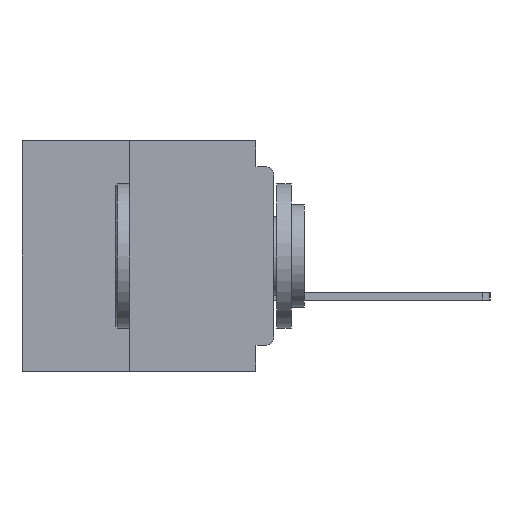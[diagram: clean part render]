
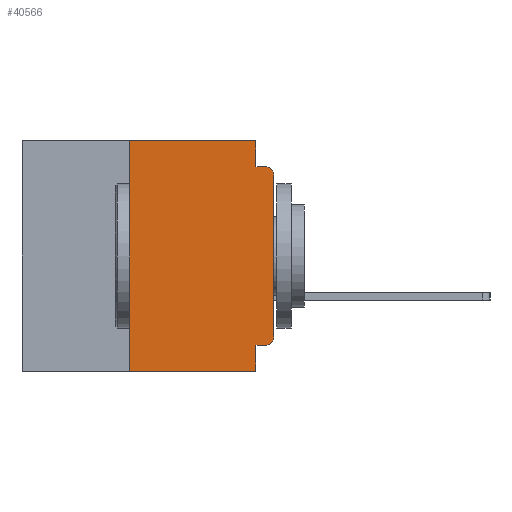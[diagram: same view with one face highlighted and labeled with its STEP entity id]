
A CAD part, left-side view. The second image highlights one B-rep face of the part: STEP entity #40566.
In plain terms, the highlighted planar face has unit normal (-1, 0, 0).
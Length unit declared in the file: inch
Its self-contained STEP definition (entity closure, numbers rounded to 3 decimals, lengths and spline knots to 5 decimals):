
#338 = VECTOR ( 'NONE', #13728, 39.37008 ) ;
#864 = CARTESIAN_POINT ( 'NONE',  ( 0., 0.015, -0.06 ) ) ;
#942 = FACE_OUTER_BOUND ( 'NONE', #18045, .T. ) ;
#963 = EDGE_CURVE ( 'NONE', #47826, #32119, #23893, .T. ) ;
#2531 = CARTESIAN_POINT ( 'NONE',  ( 0., 0.437, -0.4 ) ) ;
#3249 = VECTOR ( 'NONE', #39282, 39.37008 ) ;
#3301 = DIRECTION ( 'NONE',  ( -1., 0., 0. ) ) ;
#3614 = VECTOR ( 'NONE', #4385, 39.37008 ) ;
#4385 = DIRECTION ( 'NONE',  ( 0., 0., 1. ) ) ;
#4630 = LINE ( 'NONE', #17301, #3249 ) ;
#5365 = DIRECTION ( 'NONE',  ( 0., 0., -1. ) ) ;
#6718 = DIRECTION ( 'NONE',  ( 0., 0., 1. ) ) ;
#7392 = VECTOR ( 'NONE', #6718, 39.37008 ) ;
#7711 = EDGE_CURVE ( 'NONE', #27300, #34695, #30840, .T. ) ;
#8021 = DIRECTION ( 'NONE',  ( 0., -1., 0. ) ) ;
#8273 = VECTOR ( 'NONE', #14471, 39.37008 ) ;
#8726 = ORIENTED_EDGE ( 'NONE', *, *, #27425, .F. ) ;
#9254 = CARTESIAN_POINT ( 'NONE',  ( 0., 0.031, -0.045 ) ) ;
#9965 = CARTESIAN_POINT ( 'NONE',  ( 0., 0.437, 0. ) ) ;
#11628 = CARTESIAN_POINT ( 'NONE',  ( 0., 0.015, -0.045 ) ) ;
#11680 = DIRECTION ( 'NONE',  ( 0., -1., 0. ) ) ;
#12829 = CARTESIAN_POINT ( 'NONE',  ( 0., 0.25, 0. ) ) ;
#13066 = EDGE_CURVE ( 'NONE', #34695, #35308, #22881, .T. ) ;
#13728 = DIRECTION ( 'NONE',  ( 0., 0., -1. ) ) ;
#14253 = CARTESIAN_POINT ( 'NONE',  ( 0., 0.031, 0. ) ) ;
#14471 = DIRECTION ( 'NONE',  ( 0., -1., 0. ) ) ;
#14612 = EDGE_CURVE ( 'NONE', #47579, #37729, #56716, .T. ) ;
#15073 = VECTOR ( 'NONE', #8021, 39.37008 ) ;
#15837 = EDGE_CURVE ( 'NONE', #28583, #47826, #28098, .T. ) ;
#16372 = CARTESIAN_POINT ( 'NONE',  ( 0., 0., -0.06 ) ) ;
#17301 = CARTESIAN_POINT ( 'NONE',  ( 0., 0., -0.355 ) ) ;
#17964 = CARTESIAN_POINT ( 'NONE',  ( 0., 0., -0.34 ) ) ;
#18045 = EDGE_LOOP ( 'NONE', ( #38471, #51390, #8726, #32618, #43562, #37727, #55555, #26752, #25667, #31769 ) ) ;
#19613 = LINE ( 'NONE', #56816, #3614 ) ;
#20545 = CARTESIAN_POINT ( 'NONE',  ( 0., 0.015, -0.355 ) ) ;
#20630 = VECTOR ( 'NONE', #51260, 39.37008 ) ;
#20750 = CARTESIAN_POINT ( 'NONE',  ( 0., 0.031, -0.4 ) ) ;
#21946 = CARTESIAN_POINT ( 'NONE',  ( 0., 0.031, 0. ) ) ;
#22881 = CIRCLE ( 'NONE', #35329, 0.015 ) ;
#23310 = DIRECTION ( 'NONE',  ( 1., 0., 0. ) ) ;
#23893 = LINE ( 'NONE', #14253, #338 ) ;
#25667 = ORIENTED_EDGE ( 'NONE', *, *, #39037, .F. ) ;
#26526 = VERTEX_POINT ( 'NONE', #20545 ) ;
#26752 = ORIENTED_EDGE ( 'NONE', *, *, #14612, .F. ) ;
#27300 = VERTEX_POINT ( 'NONE', #17964 ) ;
#27425 = EDGE_CURVE ( 'NONE', #32119, #35308, #33122, .T. ) ;
#28098 = LINE ( 'NONE', #30004, #15073 ) ;
#28487 = EDGE_CURVE ( 'NONE', #26526, #27300, #35042, .T. ) ;
#28583 = VERTEX_POINT ( 'NONE', #12829 ) ;
#29053 = LINE ( 'NONE', #2531, #52221 ) ;
#29731 = CARTESIAN_POINT ( 'NONE',  ( 0., 0.015, -0.34 ) ) ;
#30004 = CARTESIAN_POINT ( 'NONE',  ( 0., 0.437, 0. ) ) ;
#30840 = LINE ( 'NONE', #33121, #7392 ) ;
#31769 = ORIENTED_EDGE ( 'NONE', *, *, #28487, .T. ) ;
#31770 = DIRECTION ( 'NONE',  ( -1., 0., 0. ) ) ;
#31912 = PLANE ( 'NONE',  #46467 ) ;
#32119 = VERTEX_POINT ( 'NONE', #9254 ) ;
#32618 = ORIENTED_EDGE ( 'NONE', *, *, #963, .F. ) ;
#33121 = CARTESIAN_POINT ( 'NONE',  ( 0., 0., 0. ) ) ;
#33122 = LINE ( 'NONE', #45072, #8273 ) ;
#34171 = DIRECTION ( 'NONE',  ( 0., 0., -1. ) ) ;
#34695 = VERTEX_POINT ( 'NONE', #16372 ) ;
#35042 = CIRCLE ( 'NONE', #49812, 0.015 ) ;
#35308 = VERTEX_POINT ( 'NONE', #11628 ) ;
#35329 = AXIS2_PLACEMENT_3D ( 'NONE', #864, #31770, #5365 ) ;
#37727 = ORIENTED_EDGE ( 'NONE', *, *, #45686, .F. ) ;
#37729 = VERTEX_POINT ( 'NONE', #42396 ) ;
#38471 = ORIENTED_EDGE ( 'NONE', *, *, #7711, .T. ) ;
#39037 = EDGE_CURVE ( 'NONE', #26526, #47579, #4630, .T. ) ;
#39282 = DIRECTION ( 'NONE',  ( 0., 1., 0. ) ) ;
#40566 = ADVANCED_FACE ( 'NONE', ( #942 ), #31912, .F. ) ;
#41871 = VERTEX_POINT ( 'NONE', #55310 ) ;
#42396 = CARTESIAN_POINT ( 'NONE',  ( 0., 0.031, -0.4 ) ) ;
#43562 = ORIENTED_EDGE ( 'NONE', *, *, #15837, .F. ) ;
#45072 = CARTESIAN_POINT ( 'NONE',  ( 0., 0., -0.045 ) ) ;
#45686 = EDGE_CURVE ( 'NONE', #41871, #28583, #19613, .T. ) ;
#46467 = AXIS2_PLACEMENT_3D ( 'NONE', #9965, #23310, #53755 ) ;
#46666 = EDGE_CURVE ( 'NONE', #41871, #37729, #29053, .T. ) ;
#47579 = VERTEX_POINT ( 'NONE', #53041 ) ;
#47826 = VERTEX_POINT ( 'NONE', #21946 ) ;
#49812 = AXIS2_PLACEMENT_3D ( 'NONE', #29731, #3301, #34171 ) ;
#51260 = DIRECTION ( 'NONE',  ( 0., 0., -1. ) ) ;
#51390 = ORIENTED_EDGE ( 'NONE', *, *, #13066, .T. ) ;
#52221 = VECTOR ( 'NONE', #11680, 39.37008 ) ;
#53041 = CARTESIAN_POINT ( 'NONE',  ( 0., 0.031, -0.355 ) ) ;
#53755 = DIRECTION ( 'NONE',  ( 0., 0., -1. ) ) ;
#55310 = CARTESIAN_POINT ( 'NONE',  ( 0., 0.25, -0.4 ) ) ;
#55555 = ORIENTED_EDGE ( 'NONE', *, *, #46666, .T. ) ;
#56716 = LINE ( 'NONE', #20750, #20630 ) ;
#56816 = CARTESIAN_POINT ( 'NONE',  ( 0., 0.25, -0.4 ) ) ;
